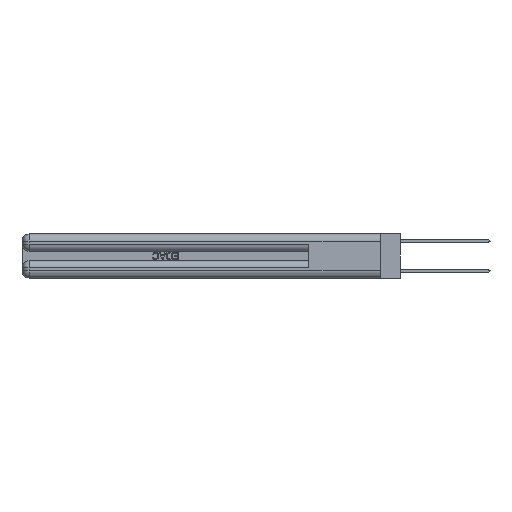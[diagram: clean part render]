
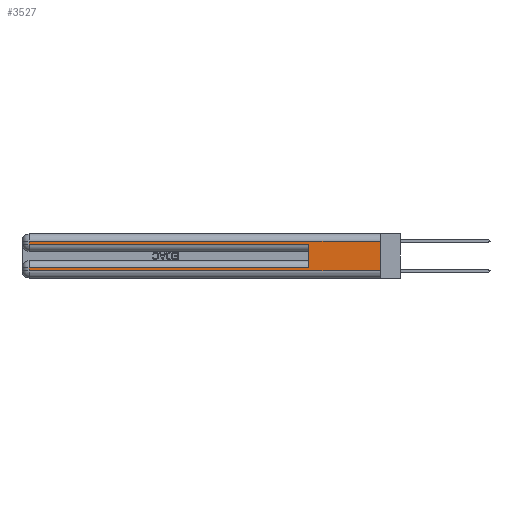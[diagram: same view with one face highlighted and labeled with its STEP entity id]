
A CAD part, left-side view. The second image highlights one B-rep face of the part: STEP entity #3527.
In plain terms, the highlighted planar face has unit normal (-1, 0, 0).
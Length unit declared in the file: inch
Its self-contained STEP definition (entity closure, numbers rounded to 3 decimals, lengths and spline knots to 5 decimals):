
#730 = DIRECTION ( 'NONE',  ( 0., -1., 0. ) ) ;
#840 = CARTESIAN_POINT ( 'NONE',  ( 0., 2.94, 0.31 ) ) ;
#918 = DIRECTION ( 'NONE',  ( 0., 0., -1. ) ) ;
#3527 = ADVANCED_FACE ( 'NONE', ( #4792 ), #20269, .F. ) ;
#4092 = VECTOR ( 'NONE', #30686, 39.37008 ) ;
#4348 = VECTOR ( 'NONE', #918, 39.37008 ) ;
#4684 = VECTOR ( 'NONE', #11092, 39.37008 ) ;
#4746 = CARTESIAN_POINT ( 'NONE',  ( 0., 0., 0.06 ) ) ;
#4792 = FACE_OUTER_BOUND ( 'NONE', #6024, .T. ) ;
#5524 = CARTESIAN_POINT ( 'NONE',  ( 0., 0., 0.085 ) ) ;
#6024 = EDGE_LOOP ( 'NONE', ( #18461, #26606, #12331, #32378, #29067, #8608, #26877, #35096 ) ) ;
#6323 = CARTESIAN_POINT ( 'NONE',  ( 0., 0., 0.285 ) ) ;
#6408 = CARTESIAN_POINT ( 'NONE',  ( 0., 2.94, 0.085 ) ) ;
#7434 = VERTEX_POINT ( 'NONE', #20860 ) ;
#7487 = DIRECTION ( 'NONE',  ( 0., -1., 0. ) ) ;
#7529 = VERTEX_POINT ( 'NONE', #21225 ) ;
#8286 = VECTOR ( 'NONE', #7487, 39.37008 ) ;
#8608 = ORIENTED_EDGE ( 'NONE', *, *, #9564, .T. ) ;
#9286 = DIRECTION ( 'NONE',  ( 1., 0., 0. ) ) ;
#9564 = EDGE_CURVE ( 'NONE', #24974, #31470, #26737, .T. ) ;
#10114 = VECTOR ( 'NONE', #21389, 39.37008 ) ;
#10459 = LINE ( 'NONE', #6323, #31684 ) ;
#10661 = DIRECTION ( 'NONE',  ( 0., 0., -1. ) ) ;
#11092 = DIRECTION ( 'NONE',  ( 0., 1., 0. ) ) ;
#11396 = EDGE_CURVE ( 'NONE', #29844, #7434, #23603, .T. ) ;
#12331 = ORIENTED_EDGE ( 'NONE', *, *, #21627, .T. ) ;
#14742 = CARTESIAN_POINT ( 'NONE',  ( 0., 2.94, 0.37 ) ) ;
#15043 = VECTOR ( 'NONE', #10661, 39.37008 ) ;
#15919 = LINE ( 'NONE', #30014, #15043 ) ;
#17278 = VERTEX_POINT ( 'NONE', #31511 ) ;
#18461 = ORIENTED_EDGE ( 'NONE', *, *, #11396, .F. ) ;
#19307 = VERTEX_POINT ( 'NONE', #840 ) ;
#20269 = PLANE ( 'NONE',  #26844 ) ;
#20449 = CARTESIAN_POINT ( 'NONE',  ( 0., 0.6, 0.085 ) ) ;
#20860 = CARTESIAN_POINT ( 'NONE',  ( 0., 0., 0.06 ) ) ;
#21225 = CARTESIAN_POINT ( 'NONE',  ( 0., 0.6, 0.285 ) ) ;
#21389 = DIRECTION ( 'NONE',  ( 0., 1., 0. ) ) ;
#21627 = EDGE_CURVE ( 'NONE', #19307, #30395, #15919, .T. ) ;
#21998 = DIRECTION ( 'NONE',  ( 0., 0., -1. ) ) ;
#22319 = CARTESIAN_POINT ( 'NONE',  ( 0., 0.6, 0.145 ) ) ;
#23603 = LINE ( 'NONE', #24758, #29236 ) ;
#23901 = EDGE_CURVE ( 'NONE', #29844, #19307, #31345, .T. ) ;
#23905 = LINE ( 'NONE', #4746, #8286 ) ;
#24758 = CARTESIAN_POINT ( 'NONE',  ( 0., 0., 0.37 ) ) ;
#24888 = EDGE_CURVE ( 'NONE', #30395, #7529, #10459, .T. ) ;
#24974 = VERTEX_POINT ( 'NONE', #20449 ) ;
#25532 = EDGE_CURVE ( 'NONE', #31470, #17278, #33801, .T. ) ;
#25836 = CARTESIAN_POINT ( 'NONE',  ( 0., 0., 0.37 ) ) ;
#26137 = LINE ( 'NONE', #22319, #4092 ) ;
#26156 = CARTESIAN_POINT ( 'NONE',  ( 0., 2.94, 0.285 ) ) ;
#26606 = ORIENTED_EDGE ( 'NONE', *, *, #23901, .T. ) ;
#26737 = LINE ( 'NONE', #5524, #4684 ) ;
#26844 = AXIS2_PLACEMENT_3D ( 'NONE', #25836, #9286, #28632 ) ;
#26877 = ORIENTED_EDGE ( 'NONE', *, *, #25532, .T. ) ;
#28632 = DIRECTION ( 'NONE',  ( 0., 0., -1. ) ) ;
#29067 = ORIENTED_EDGE ( 'NONE', *, *, #30132, .F. ) ;
#29236 = VECTOR ( 'NONE', #21998, 39.37008 ) ;
#29844 = VERTEX_POINT ( 'NONE', #32045 ) ;
#30014 = CARTESIAN_POINT ( 'NONE',  ( 0., 2.94, 0.37 ) ) ;
#30132 = EDGE_CURVE ( 'NONE', #24974, #7529, #26137, .T. ) ;
#30395 = VERTEX_POINT ( 'NONE', #26156 ) ;
#30686 = DIRECTION ( 'NONE',  ( 0., 0., 1. ) ) ;
#31345 = LINE ( 'NONE', #35200, #10114 ) ;
#31470 = VERTEX_POINT ( 'NONE', #6408 ) ;
#31511 = CARTESIAN_POINT ( 'NONE',  ( 0., 2.94, 0.06 ) ) ;
#31684 = VECTOR ( 'NONE', #730, 39.37008 ) ;
#32045 = CARTESIAN_POINT ( 'NONE',  ( 0., 0., 0.31 ) ) ;
#32378 = ORIENTED_EDGE ( 'NONE', *, *, #24888, .T. ) ;
#33801 = LINE ( 'NONE', #14742, #4348 ) ;
#34694 = EDGE_CURVE ( 'NONE', #17278, #7434, #23905, .T. ) ;
#35096 = ORIENTED_EDGE ( 'NONE', *, *, #34694, .T. ) ;
#35200 = CARTESIAN_POINT ( 'NONE',  ( 0., 0., 0.31 ) ) ;
